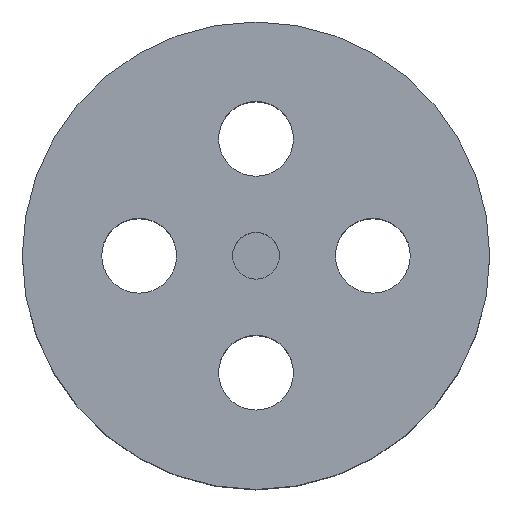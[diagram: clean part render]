
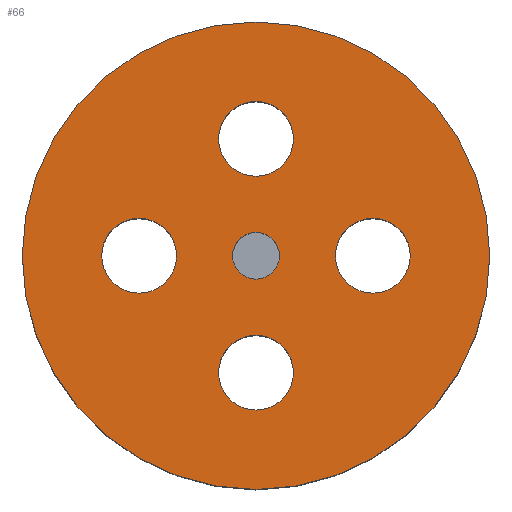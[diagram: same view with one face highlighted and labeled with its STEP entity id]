
A CAD part, top view. The second image highlights one B-rep face of the part: STEP entity #66.
In plain terms, the highlighted planar face has unit normal (0, 0, 1).
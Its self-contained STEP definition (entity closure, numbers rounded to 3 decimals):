
#9 = FACE_BOUND ( 'NONE', #115, .T. ) ;
#11 = FACE_BOUND ( 'NONE', #72, .T. ) ;
#13 = FACE_BOUND ( 'NONE', #98, .T. ) ;
#14 = FACE_BOUND ( 'NONE', #103, .T. ) ;
#17 = CIRCLE ( 'NONE', #775, 4. ) ;
#34 = CIRCLE ( 'NONE', #776, 4. ) ;
#66 = ADVANCED_FACE ( 'NONE', ( #9, #14, #940, #11, #13, #888 ), #654, .T. ) ;
#72 = EDGE_LOOP ( 'NONE', ( #411, #426 ) ) ;
#74 = VERTEX_POINT ( 'NONE', #633 ) ;
#85 = EDGE_LOOP ( 'NONE', ( #342, #452 ) ) ;
#98 = EDGE_LOOP ( 'NONE', ( #431, #430 ) ) ;
#102 = EDGE_LOOP ( 'NONE', ( #347, #327 ) ) ;
#103 = EDGE_LOOP ( 'NONE', ( #405, #415 ) ) ;
#115 = EDGE_LOOP ( 'NONE', ( #417, #383 ) ) ;
#319 = VERTEX_POINT ( 'NONE', #609 ) ;
#320 = VERTEX_POINT ( 'NONE', #605 ) ;
#322 = VERTEX_POINT ( 'NONE', #603 ) ;
#325 = VERTEX_POINT ( 'NONE', #601 ) ;
#327 = ORIENTED_EDGE ( 'NONE', *, *, #717, .T. ) ;
#331 = VERTEX_POINT ( 'NONE', #584 ) ;
#342 = ORIENTED_EDGE ( 'NONE', *, *, #718, .T. ) ;
#347 = ORIENTED_EDGE ( 'NONE', *, *, #697, .T. ) ;
#383 = ORIENTED_EDGE ( 'NONE', *, *, #698, .T. ) ;
#385 = VERTEX_POINT ( 'NONE', #569 ) ;
#394 = VERTEX_POINT ( 'NONE', #557 ) ;
#396 = VERTEX_POINT ( 'NONE', #555 ) ;
#397 = VERTEX_POINT ( 'NONE', #546 ) ;
#399 = VERTEX_POINT ( 'NONE', #544 ) ;
#405 = ORIENTED_EDGE ( 'NONE', *, *, #684, .T. ) ;
#408 = VERTEX_POINT ( 'NONE', #537 ) ;
#411 = ORIENTED_EDGE ( 'NONE', *, *, #713, .F. ) ;
#415 = ORIENTED_EDGE ( 'NONE', *, *, #716, .T. ) ;
#417 = ORIENTED_EDGE ( 'NONE', *, *, #708, .T. ) ;
#426 = ORIENTED_EDGE ( 'NONE', *, *, #710, .F. ) ;
#430 = ORIENTED_EDGE ( 'NONE', *, *, #714, .T. ) ;
#431 = ORIENTED_EDGE ( 'NONE', *, *, #682, .T. ) ;
#452 = ORIENTED_EDGE ( 'NONE', *, *, #694, .T. ) ;
#495 = DIRECTION ( 'NONE',  ( 1., 0., 0. ) ) ;
#496 = DIRECTION ( 'NONE',  ( 0., 0., 1. ) ) ;
#497 = CARTESIAN_POINT ( 'NONE',  ( 0., 0., 30. ) ) ;
#501 = DIRECTION ( 'NONE',  ( 1., 0., 0. ) ) ;
#502 = DIRECTION ( 'NONE',  ( 0., 0., -1. ) ) ;
#503 = CARTESIAN_POINT ( 'NONE',  ( 12.5, 0., 30. ) ) ;
#507 = DIRECTION ( 'NONE',  ( 1., 0., 0. ) ) ;
#509 = DIRECTION ( 'NONE',  ( 0., 0., -1. ) ) ;
#510 = CARTESIAN_POINT ( 'NONE',  ( 0., -12.5, 30. ) ) ;
#521 = DIRECTION ( 'NONE',  ( 1., 0., 0. ) ) ;
#522 = DIRECTION ( 'NONE',  ( 0., 0., -1. ) ) ;
#523 = CARTESIAN_POINT ( 'NONE',  ( -12.5, 0., 30. ) ) ;
#528 = DIRECTION ( 'NONE',  ( 1., 0., 0. ) ) ;
#529 = DIRECTION ( 'NONE',  ( 0., 0., 1. ) ) ;
#531 = CARTESIAN_POINT ( 'NONE',  ( 0., 0., 30. ) ) ;
#537 = CARTESIAN_POINT ( 'NONE',  ( 16.5, 0., 30. ) ) ;
#538 = DIRECTION ( 'NONE',  ( 1., 0., 0. ) ) ;
#539 = DIRECTION ( 'NONE',  ( 0., 0., 1. ) ) ;
#540 = CARTESIAN_POINT ( 'NONE',  ( 0., 0., 30. ) ) ;
#544 = CARTESIAN_POINT ( 'NONE',  ( 4., 12.5, 30. ) ) ;
#546 = CARTESIAN_POINT ( 'NONE',  ( 8.5, 0., 30. ) ) ;
#548 = DIRECTION ( 'NONE',  ( 1., 0., 0. ) ) ;
#549 = DIRECTION ( 'NONE',  ( 0., 0., -1. ) ) ;
#553 = CARTESIAN_POINT ( 'NONE',  ( 0., 12.5, 30. ) ) ;
#555 = CARTESIAN_POINT ( 'NONE',  ( -4., 12.5, 30. ) ) ;
#557 = CARTESIAN_POINT ( 'NONE',  ( -4., -12.5, 30. ) ) ;
#569 = CARTESIAN_POINT ( 'NONE',  ( 4., -12.5, 30. ) ) ;
#584 = CARTESIAN_POINT ( 'NONE',  ( 2.5, 0., 30. ) ) ;
#586 = DIRECTION ( 'NONE',  ( 1., 0., 0. ) ) ;
#587 = DIRECTION ( 'NONE',  ( 0., 0., -1. ) ) ;
#588 = CARTESIAN_POINT ( 'NONE',  ( 0., 12.5, 30. ) ) ;
#592 = DIRECTION ( 'NONE',  ( 1., 0., 0. ) ) ;
#593 = DIRECTION ( 'NONE',  ( 0., 0., -1. ) ) ;
#594 = CARTESIAN_POINT ( 'NONE',  ( 12.5, 0., 30. ) ) ;
#601 = CARTESIAN_POINT ( 'NONE',  ( 25., 0., 30. ) ) ;
#603 = CARTESIAN_POINT ( 'NONE',  ( -2.5, 0., 30. ) ) ;
#605 = CARTESIAN_POINT ( 'NONE',  ( -25., 0., 30. ) ) ;
#608 = DIRECTION ( 'NONE',  ( 1., 0., 0. ) ) ;
#609 = CARTESIAN_POINT ( 'NONE',  ( -16.5, 0., 30. ) ) ;
#610 = DIRECTION ( 'NONE',  ( 0., 0., 1. ) ) ;
#611 = CARTESIAN_POINT ( 'NONE',  ( 0., 0., 30. ) ) ;
#633 = CARTESIAN_POINT ( 'NONE',  ( -8.5, 0., 30. ) ) ;
#644 = DIRECTION ( 'NONE',  ( 1., 0., 0. ) ) ;
#646 = DIRECTION ( 'NONE',  ( 0., 0., -1. ) ) ;
#647 = CARTESIAN_POINT ( 'NONE',  ( 0., -12.5, 30. ) ) ;
#654 = PLANE ( 'NONE',  #767 ) ;
#656 = DIRECTION ( 'NONE',  ( 1., 0., 0. ) ) ;
#657 = CARTESIAN_POINT ( 'NONE',  ( 0., 0., 30. ) ) ;
#659 = DIRECTION ( 'NONE',  ( 0., 0., -1. ) ) ;
#660 = CARTESIAN_POINT ( 'NONE',  ( -12.5, 0., 30. ) ) ;
#662 = DIRECTION ( 'NONE',  ( 1., 0., 0. ) ) ;
#670 = DIRECTION ( 'NONE',  ( 0., 0., 1. ) ) ;
#682 = EDGE_CURVE ( 'NONE', #74, #319, #17, .T. ) ;
#684 = EDGE_CURVE ( 'NONE', #385, #394, #34, .T. ) ;
#694 = EDGE_CURVE ( 'NONE', #325, #320, #862, .T. ) ;
#697 = EDGE_CURVE ( 'NONE', #408, #397, #880, .T. ) ;
#698 = EDGE_CURVE ( 'NONE', #396, #399, #870, .T. ) ;
#708 = EDGE_CURVE ( 'NONE', #399, #396, #817, .T. ) ;
#710 = EDGE_CURVE ( 'NONE', #322, #331, #841, .T. ) ;
#713 = EDGE_CURVE ( 'NONE', #331, #322, #869, .T. ) ;
#714 = EDGE_CURVE ( 'NONE', #319, #74, #878, .T. ) ;
#716 = EDGE_CURVE ( 'NONE', #394, #385, #845, .T. ) ;
#717 = EDGE_CURVE ( 'NONE', #397, #408, #822, .T. ) ;
#718 = EDGE_CURVE ( 'NONE', #320, #325, #830, .T. ) ;
#767 = AXIS2_PLACEMENT_3D ( 'NONE', #657, #670, #662 ) ;
#775 = AXIS2_PLACEMENT_3D ( 'NONE', #660, #659, #656 ) ;
#776 = AXIS2_PLACEMENT_3D ( 'NONE', #647, #646, #644 ) ;
#779 = AXIS2_PLACEMENT_3D ( 'NONE', #611, #610, #608 ) ;
#781 = AXIS2_PLACEMENT_3D ( 'NONE', #594, #593, #592 ) ;
#782 = AXIS2_PLACEMENT_3D ( 'NONE', #588, #587, #586 ) ;
#786 = AXIS2_PLACEMENT_3D ( 'NONE', #553, #549, #548 ) ;
#787 = AXIS2_PLACEMENT_3D ( 'NONE', #540, #539, #538 ) ;
#788 = AXIS2_PLACEMENT_3D ( 'NONE', #531, #529, #528 ) ;
#789 = AXIS2_PLACEMENT_3D ( 'NONE', #523, #522, #521 ) ;
#791 = AXIS2_PLACEMENT_3D ( 'NONE', #510, #509, #507 ) ;
#792 = AXIS2_PLACEMENT_3D ( 'NONE', #503, #502, #501 ) ;
#793 = AXIS2_PLACEMENT_3D ( 'NONE', #497, #496, #495 ) ;
#817 = CIRCLE ( 'NONE', #786, 4. ) ;
#822 = CIRCLE ( 'NONE', #792, 4. ) ;
#830 = CIRCLE ( 'NONE', #793, 25. ) ;
#841 = CIRCLE ( 'NONE', #787, 2.5 ) ;
#845 = CIRCLE ( 'NONE', #791, 4. ) ;
#862 = CIRCLE ( 'NONE', #779, 25. ) ;
#869 = CIRCLE ( 'NONE', #788, 2.5 ) ;
#870 = CIRCLE ( 'NONE', #782, 4. ) ;
#878 = CIRCLE ( 'NONE', #789, 4. ) ;
#880 = CIRCLE ( 'NONE', #781, 4. ) ;
#888 = FACE_BOUND ( 'NONE', #102, .T. ) ;
#940 = FACE_OUTER_BOUND ( 'NONE', #85, .T. ) ;
